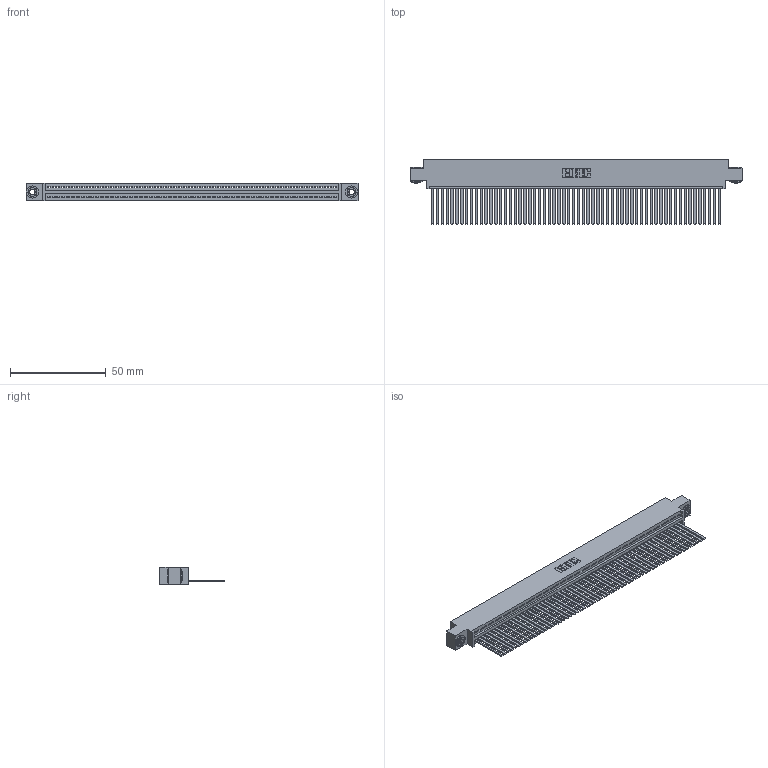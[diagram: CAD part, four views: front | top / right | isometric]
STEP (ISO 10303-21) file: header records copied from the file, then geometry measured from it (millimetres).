
FILE_DESCRIPTION (( 'STEP AP203' ), '1' );
FILE_NAME ('395-060-544-603.STEP', '2019-10-24T13:08:16', ( '' ), ( '' ), 'SwSTEP 2.0', 'SolidWorks 2016', '' );
FILE_SCHEMA (( 'CONFIG_CONTROL_DESIGN' ));
Length unit declared in the file: inch
Products named in the file (4): 345-250-002_345-250-002-102; 395-060-544-603; 345-292-001_345-293-144; 345 Part_0.170 Offset - 0.156 Dia-TH
Assembly tree (63 placements, depth 2):
  395-060-544-603
    345 Part_0.170 Offset - 0.156 Dia-TH
    345-292-001_345-293-144  x60
    345-250-002_345-250-002-102  x2
Bounding box: 173.61 x 33.96 x 9.4 mm (x, y, z)
Volume: 17237.9 mm3; surface area: 25579.4 mm2
Topology: 63 solids, 63 shells, 3288 faces, 9909 edges, 6522 vertices
Faces by surface type: plane 2254, cylinder 1026, cone 8
Entity records: 43332 total; most frequent: CARTESIAN_POINT 7483, ORIENTED_EDGE 7470, DIRECTION 6537, EDGE_CURVE 3735, VECTOR 3343, LINE 3343, VERTEX_POINT 2486, AXIS2_PLACEMENT_3D 1597
